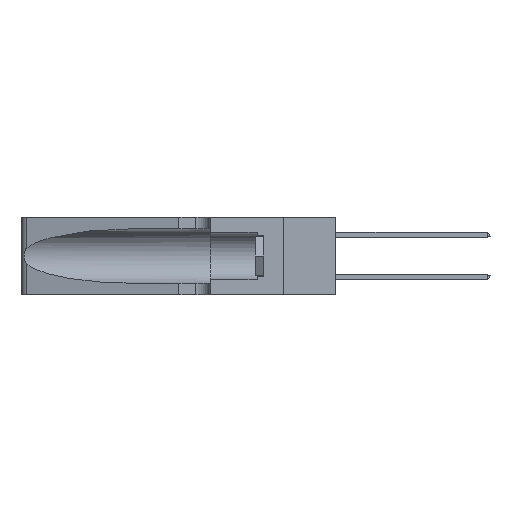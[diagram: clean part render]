
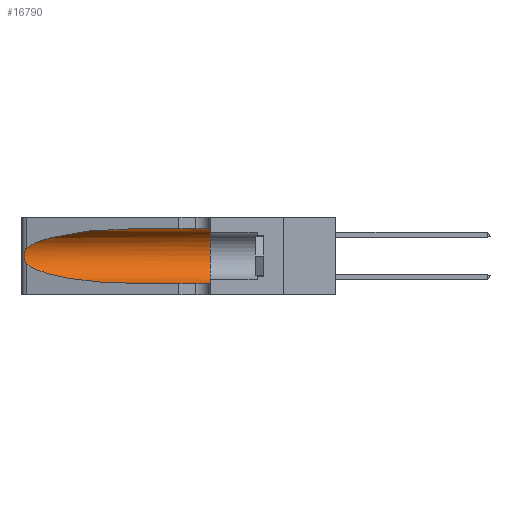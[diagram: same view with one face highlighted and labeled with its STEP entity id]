
A CAD part, left-side view. The second image highlights one B-rep face of the part: STEP entity #16790.
In plain terms, the highlighted cylindrical face has radius 3.308 mm (diameter 6.617 mm), a partial arc.
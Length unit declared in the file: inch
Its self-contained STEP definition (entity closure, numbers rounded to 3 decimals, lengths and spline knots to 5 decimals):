
#719 = DIRECTION ( 'NONE',  ( 0., 0., -1. ) ) ;
#1096 = CARTESIAN_POINT ( 'NONE',  ( 0.25639, 1.23184, 0.21858 ) ) ;
#1278 = CYLINDRICAL_SURFACE ( 'NONE', #10329, 0.13025 ) ;
#1648 =( BOUNDED_CURVE ( )  B_SPLINE_CURVE ( 3, ( #4884, #12128, #13881, #3116 ),
 .UNSPECIFIED., .F., .T. ) 
 B_SPLINE_CURVE_WITH_KNOTS ( ( 4, 4 ),
 ( 3.44316, 4.71239 ),
 .UNSPECIFIED. ) 
 CURVE ( )  GEOMETRIC_REPRESENTATION_ITEM ( )  RATIONAL_B_SPLINE_CURVE ( ( 1., 0.87, 0.87, 1. ) ) 
 REPRESENTATION_ITEM ( '' )  );
#2083 =( BOUNDED_CURVE ( )  B_SPLINE_CURVE ( 3, ( #10109, #13581, #20691, #22483 ),
 .UNSPECIFIED., .F., .F. ) 
 B_SPLINE_CURVE_WITH_KNOTS ( ( 4, 4 ),
 ( 1.5708, 2.84003 ),
 .UNSPECIFIED. ) 
 CURVE ( )  GEOMETRIC_REPRESENTATION_ITEM ( )  RATIONAL_B_SPLINE_CURVE ( ( 1., 0.87, 0.87, 1. ) ) 
 REPRESENTATION_ITEM ( '' )  );
#2824 = CARTESIAN_POINT ( 'NONE',  ( 0.1305, 1.61858, 0.05475 ) ) ;
#2883 = CARTESIAN_POINT ( 'NONE',  ( 0.25555, 1.22994, 0.2215 ) ) ;
#2964 = CARTESIAN_POINT ( 'NONE',  ( 0.25854, 1.2359, 0.20912 ) ) ;
#3116 = CARTESIAN_POINT ( 'NONE',  ( 0.1305, 0.72297, 0.05475 ) ) ;
#3555 = VERTEX_POINT ( 'NONE', #12226 ) ;
#4105 = EDGE_CURVE ( 'NONE', #5337, #10882, #2083, .T. ) ;
#4674 = DIRECTION ( 'NONE',  ( 0., -1., 0. ) ) ;
#4809 = CARTESIAN_POINT ( 'NONE',  ( 0.26075, 1.23896, 0.19203 ) ) ;
#4884 = CARTESIAN_POINT ( 'NONE',  ( 0.25487, 1.22718, 0.14631 ) ) ;
#5337 = VERTEX_POINT ( 'NONE', #17819 ) ;
#6073 = LINE ( 'NONE', #2824, #14425 ) ;
#6089 = DIRECTION ( 'NONE',  ( 0., -1., 0. ) ) ;
#6420 = EDGE_LOOP ( 'NONE', ( #7964, #21832, #17433, #8436, #18857, #14259 ) ) ;
#6624 = VERTEX_POINT ( 'NONE', #15894 ) ;
#6651 = CARTESIAN_POINT ( 'NONE',  ( 0.26017, 1.23833, 0.17102 ) ) ;
#6953 = EDGE_CURVE ( 'NONE', #5337, #13528, #13406, .T. ) ;
#7964 = ORIENTED_EDGE ( 'NONE', *, *, #4105, .T. ) ;
#8069 = EDGE_CURVE ( 'NONE', #18194, #6624, #6073, .T. ) ;
#8392 = CARTESIAN_POINT ( 'NONE',  ( 0.25487, 1.22718, 0.22369 ) ) ;
#8436 = ORIENTED_EDGE ( 'NONE', *, *, #8069, .T. ) ;
#8467 = CARTESIAN_POINT ( 'NONE',  ( 0.25789, 1.23486, 0.15765 ) ) ;
#8873 = EDGE_CURVE ( 'NONE', #3555, #18194, #1648, .T. ) ;
#9200 = DIRECTION ( 'NONE',  ( 0., 1., 0. ) ) ;
#9728 = EDGE_CURVE ( 'NONE', #13528, #6624, #19604, .T. ) ;
#10109 = CARTESIAN_POINT ( 'NONE',  ( 0.1305, 0.72297, 0.31525 ) ) ;
#10281 = CARTESIAN_POINT ( 'NONE',  ( 0.25555, 1.22993, 0.14849 ) ) ;
#10329 = AXIS2_PLACEMENT_3D ( 'NONE', #13399, #16831, #719 ) ;
#10882 = VERTEX_POINT ( 'NONE', #11513 ) ;
#10981 = FACE_OUTER_BOUND ( 'NONE', #6420, .T. ) ;
#11396 = B_SPLINE_CURVE_WITH_KNOTS ( 'NONE', 3,
 ( #8392, #2883, #1096, #13736, #2964, #15510, #4809, #17266, #6651, #19073, #8467, #20854, #10281, #22638 ),
 .UNSPECIFIED., .F., .F.,
 ( 4, 2, 2, 2, 2, 2, 4 ),
 ( 0., 0.00027, 0.00053, 0.00107, 0.0016, 0.00187, 0.00214 ),
 .UNSPECIFIED. ) ;
#11513 = CARTESIAN_POINT ( 'NONE',  ( 0.25487, 1.22718, 0.22369 ) ) ;
#11888 = CARTESIAN_POINT ( 'NONE',  ( 0.1305, 0.72297, 0.05475 ) ) ;
#12128 = CARTESIAN_POINT ( 'NONE',  ( 0.2373, 1.15595, 0.08982 ) ) ;
#12226 = CARTESIAN_POINT ( 'NONE',  ( 0.25487, 1.22718, 0.14631 ) ) ;
#12306 = VECTOR ( 'NONE', #6089, 39.37008 ) ;
#13399 = CARTESIAN_POINT ( 'NONE',  ( 0.1305, 1.61858, 0.185 ) ) ;
#13406 = LINE ( 'NONE', #22099, #12306 ) ;
#13528 = VERTEX_POINT ( 'NONE', #15607 ) ;
#13581 = CARTESIAN_POINT ( 'NONE',  ( 0.18966, 0.96281, 0.31525 ) ) ;
#13736 = CARTESIAN_POINT ( 'NONE',  ( 0.25787, 1.23484, 0.2124 ) ) ;
#13881 = CARTESIAN_POINT ( 'NONE',  ( 0.18966, 0.96281, 0.05475 ) ) ;
#14259 = ORIENTED_EDGE ( 'NONE', *, *, #6953, .F. ) ;
#14425 = VECTOR ( 'NONE', #4674, 39.37008 ) ;
#15510 = CARTESIAN_POINT ( 'NONE',  ( 0.26018, 1.23835, 0.19895 ) ) ;
#15607 = CARTESIAN_POINT ( 'NONE',  ( 0.1305, 0.35, 0.31525 ) ) ;
#15894 = CARTESIAN_POINT ( 'NONE',  ( 0.1305, 0.35, 0.05475 ) ) ;
#16790 = ADVANCED_FACE ( 'NONE', ( #10981 ), #1278, .F. ) ;
#16831 = DIRECTION ( 'NONE',  ( 0., -1., 0. ) ) ;
#17266 = CARTESIAN_POINT ( 'NONE',  ( 0.26075, 1.23896, 0.178 ) ) ;
#17433 = ORIENTED_EDGE ( 'NONE', *, *, #8873, .T. ) ;
#17819 = CARTESIAN_POINT ( 'NONE',  ( 0.1305, 0.72297, 0.31525 ) ) ;
#18194 = VERTEX_POINT ( 'NONE', #11888 ) ;
#18857 = ORIENTED_EDGE ( 'NONE', *, *, #9728, .F. ) ;
#19073 = CARTESIAN_POINT ( 'NONE',  ( 0.25856, 1.23593, 0.16098 ) ) ;
#19604 = CIRCLE ( 'NONE', #22506, 0.13025 ) ;
#19795 = CARTESIAN_POINT ( 'NONE',  ( 0.1305, 0.35, 0.185 ) ) ;
#20691 = CARTESIAN_POINT ( 'NONE',  ( 0.2373, 1.15595, 0.28018 ) ) ;
#20854 = CARTESIAN_POINT ( 'NONE',  ( 0.25639, 1.23186, 0.15144 ) ) ;
#21588 = DIRECTION ( 'NONE',  ( 0., 0., 1. ) ) ;
#21832 = ORIENTED_EDGE ( 'NONE', *, *, #22156, .T. ) ;
#22099 = CARTESIAN_POINT ( 'NONE',  ( 0.1305, 1.61858, 0.31525 ) ) ;
#22156 = EDGE_CURVE ( 'NONE', #10882, #3555, #11396, .T. ) ;
#22483 = CARTESIAN_POINT ( 'NONE',  ( 0.25487, 1.22718, 0.22369 ) ) ;
#22506 = AXIS2_PLACEMENT_3D ( 'NONE', #19795, #9200, #21588 ) ;
#22638 = CARTESIAN_POINT ( 'NONE',  ( 0.25487, 1.22718, 0.14631 ) ) ;
